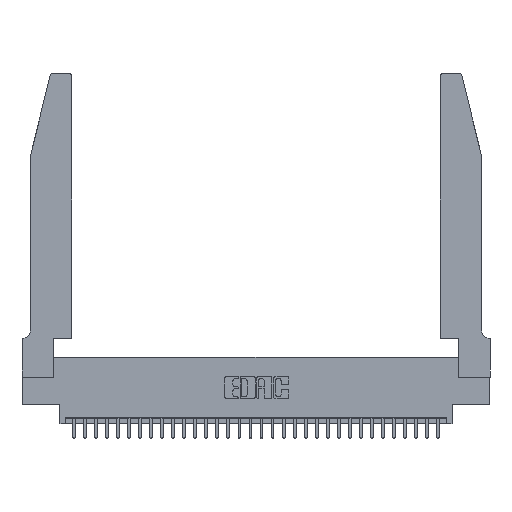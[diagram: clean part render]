
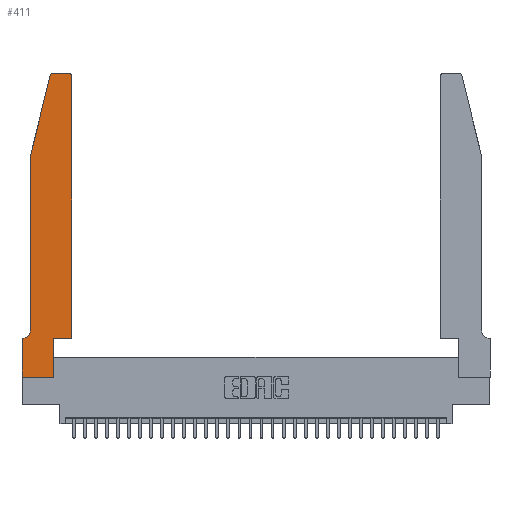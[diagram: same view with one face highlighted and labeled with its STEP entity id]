
A CAD part, top view. The second image highlights one B-rep face of the part: STEP entity #411.
In plain terms, the highlighted planar face has unit normal (0, 0, 1).
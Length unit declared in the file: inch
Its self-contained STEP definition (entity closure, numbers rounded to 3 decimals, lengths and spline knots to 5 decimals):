
#38 = ORIENTED_EDGE ( 'NONE', *, *, #1586, .T. ) ;
#411 = ADVANCED_FACE ( 'NONE', ( #4819 ), #22906, .T. ) ;
#814 = VERTEX_POINT ( 'NONE', #14764 ) ;
#944 = VECTOR ( 'NONE', #4393, 39.37008 ) ;
#1363 = CARTESIAN_POINT ( 'NONE',  ( 0., 0., 0.37 ) ) ;
#1586 = EDGE_CURVE ( 'NONE', #8249, #31456, #18300, .T. ) ;
#1672 = LINE ( 'NONE', #8475, #20260 ) ;
#2042 = ORIENTED_EDGE ( 'NONE', *, *, #30011, .T. ) ;
#2322 = CARTESIAN_POINT ( 'NONE',  ( 0.0055, 0.42, 0.37 ) ) ;
#2720 = CARTESIAN_POINT ( 'NONE',  ( 0.4505, 0.35, 0.37 ) ) ;
#2846 = ORIENTED_EDGE ( 'NONE', *, *, #5750, .T. ) ;
#3262 = ORIENTED_EDGE ( 'NONE', *, *, #23951, .T. ) ;
#3303 = VERTEX_POINT ( 'NONE', #9150 ) ;
#3480 = DIRECTION ( 'NONE',  ( 0., 1., 0. ) ) ;
#3857 = VECTOR ( 'NONE', #28769, 39.37008 ) ;
#3922 = DIRECTION ( 'NONE',  ( 0., -1., 0. ) ) ;
#4048 = ORIENTED_EDGE ( 'NONE', *, *, #29723, .T. ) ;
#4266 = AXIS2_PLACEMENT_3D ( 'NONE', #14366, #31878, #16881 ) ;
#4328 = VECTOR ( 'NONE', #3480, 39.37008 ) ;
#4393 = DIRECTION ( 'NONE',  ( 1., 0., 0. ) ) ;
#4819 = FACE_OUTER_BOUND ( 'NONE', #18458, .T. ) ;
#4869 = DIRECTION ( 'NONE',  ( -1., 0., 0. ) ) ;
#5144 = LINE ( 'NONE', #1363, #11954 ) ;
#5384 = EDGE_CURVE ( 'NONE', #3303, #18083, #32513, .T. ) ;
#5750 = EDGE_CURVE ( 'NONE', #12288, #8249, #10564, .T. ) ;
#6104 = CARTESIAN_POINT ( 'NONE',  ( 0., 0., 0.37 ) ) ;
#6639 = CARTESIAN_POINT ( 'NONE',  ( 0.2865, 0., 0.37 ) ) ;
#6648 = CARTESIAN_POINT ( 'NONE',  ( 0.0755, 0.35, 0.37 ) ) ;
#7475 = CARTESIAN_POINT ( 'NONE',  ( 0.284, 2.72, 0.37 ) ) ;
#7610 = VECTOR ( 'NONE', #21838, 39.37008 ) ;
#7743 = LINE ( 'NONE', #19524, #944 ) ;
#8249 = VERTEX_POINT ( 'NONE', #21257 ) ;
#8399 = LINE ( 'NONE', #6648, #7610 ) ;
#8475 = CARTESIAN_POINT ( 'NONE',  ( 0.2605, 2.75, 0.37 ) ) ;
#8563 = AXIS2_PLACEMENT_3D ( 'NONE', #7475, #25084, #10050 ) ;
#9035 = CARTESIAN_POINT ( 'NONE',  ( 0.4205, 2.75, 0.37 ) ) ;
#9063 = EDGE_CURVE ( 'NONE', #814, #18922, #18988, .T. ) ;
#9150 = CARTESIAN_POINT ( 'NONE',  ( 0.4505, 0.35, 0.37 ) ) ;
#9441 = LINE ( 'NONE', #22364, #11059 ) ;
#10050 = DIRECTION ( 'NONE',  ( 1., 0., 0. ) ) ;
#10564 = LINE ( 'NONE', #24123, #29731 ) ;
#10601 = VERTEX_POINT ( 'NONE', #6639 ) ;
#11059 = VECTOR ( 'NONE', #24932, 39.37008 ) ;
#11954 = VECTOR ( 'NONE', #29141, 39.37008 ) ;
#12288 = VERTEX_POINT ( 'NONE', #15922 ) ;
#13344 = VECTOR ( 'NONE', #17918, 39.37008 ) ;
#13607 = ORIENTED_EDGE ( 'NONE', *, *, #23360, .T. ) ;
#13981 = ORIENTED_EDGE ( 'NONE', *, *, #9063, .T. ) ;
#13996 = CARTESIAN_POINT ( 'NONE',  ( 0.4505, 2.72, 0.37 ) ) ;
#14155 = VERTEX_POINT ( 'NONE', #14190 ) ;
#14190 = CARTESIAN_POINT ( 'NONE',  ( 0., 0.35, 0.37 ) ) ;
#14366 = CARTESIAN_POINT ( 'NONE',  ( 0.4205, 2.72, 0.37 ) ) ;
#14764 = CARTESIAN_POINT ( 'NONE',  ( 0.284, 2.75, 0.37 ) ) ;
#15562 = ORIENTED_EDGE ( 'NONE', *, *, #19758, .T. ) ;
#15625 = AXIS2_PLACEMENT_3D ( 'NONE', #2322, #20011, #4869 ) ;
#15922 = CARTESIAN_POINT ( 'NONE',  ( 0.0755, 2., 0.37 ) ) ;
#16015 = VERTEX_POINT ( 'NONE', #28759 ) ;
#16089 = DIRECTION ( 'NONE',  ( -1., 0., 0. ) ) ;
#16842 = EDGE_CURVE ( 'NONE', #16015, #3303, #7743, .T. ) ;
#16881 = DIRECTION ( 'NONE',  ( 1., 0., 0. ) ) ;
#17330 = LINE ( 'NONE', #6104, #3857 ) ;
#17918 = DIRECTION ( 'NONE',  ( 0., 1., 0. ) ) ;
#18083 = VERTEX_POINT ( 'NONE', #13996 ) ;
#18300 = CIRCLE ( 'NONE', #15625, 0.07 ) ;
#18363 = ORIENTED_EDGE ( 'NONE', *, *, #5384, .T. ) ;
#18458 = EDGE_LOOP ( 'NONE', ( #26886, #13981, #2042, #2846, #38, #13607, #3262, #4048, #15562, #28899, #18363, #25811 ) ) ;
#18567 = DIRECTION ( 'NONE',  ( 1., 0., 0. ) ) ;
#18648 = CARTESIAN_POINT ( 'NONE',  ( 0.2865, 0.35, 0.37 ) ) ;
#18922 = VERTEX_POINT ( 'NONE', #27846 ) ;
#18952 = VERTEX_POINT ( 'NONE', #22902 ) ;
#18988 = CIRCLE ( 'NONE', #8563, 0.03 ) ;
#19524 = CARTESIAN_POINT ( 'NONE',  ( 0.4505, 0.35, 0.37 ) ) ;
#19758 = EDGE_CURVE ( 'NONE', #10601, #16015, #31110, .T. ) ;
#19877 = CARTESIAN_POINT ( 'NONE',  ( 0., 0.35, 0.37 ) ) ;
#20011 = DIRECTION ( 'NONE',  ( 0., 0., -1. ) ) ;
#20260 = VECTOR ( 'NONE', #16089, 39.37008 ) ;
#20861 = AXIS2_PLACEMENT_3D ( 'NONE', #19877, #26525, #18567 ) ;
#21257 = CARTESIAN_POINT ( 'NONE',  ( 0.0755, 0.42, 0.37 ) ) ;
#21838 = DIRECTION ( 'NONE',  ( -1., 0., 0. ) ) ;
#22364 = CARTESIAN_POINT ( 'NONE',  ( 0.0755, 2., 0.37 ) ) ;
#22424 = EDGE_CURVE ( 'NONE', #30726, #814, #1672, .T. ) ;
#22902 = CARTESIAN_POINT ( 'NONE',  ( 0., 0., 0.37 ) ) ;
#22906 = PLANE ( 'NONE',  #20861 ) ;
#23360 = EDGE_CURVE ( 'NONE', #31456, #14155, #8399, .T. ) ;
#23702 = CIRCLE ( 'NONE', #4266, 0.03 ) ;
#23951 = EDGE_CURVE ( 'NONE', #14155, #18952, #5144, .T. ) ;
#24041 = EDGE_CURVE ( 'NONE', #18083, #30726, #23702, .T. ) ;
#24123 = CARTESIAN_POINT ( 'NONE',  ( 0.0755, 2., 0.37 ) ) ;
#24592 = CARTESIAN_POINT ( 'NONE',  ( 0.0055, 0.35, 0.37 ) ) ;
#24932 = DIRECTION ( 'NONE',  ( -0.239, -0.971, 0. ) ) ;
#25084 = DIRECTION ( 'NONE',  ( 0., 0., 1. ) ) ;
#25811 = ORIENTED_EDGE ( 'NONE', *, *, #24041, .T. ) ;
#26525 = DIRECTION ( 'NONE',  ( 0., 0., 1. ) ) ;
#26886 = ORIENTED_EDGE ( 'NONE', *, *, #22424, .T. ) ;
#27846 = CARTESIAN_POINT ( 'NONE',  ( 0.25487, 2.72718, 0.37 ) ) ;
#28759 = CARTESIAN_POINT ( 'NONE',  ( 0.2865, 0.35, 0.37 ) ) ;
#28769 = DIRECTION ( 'NONE',  ( 1., 0., 0. ) ) ;
#28899 = ORIENTED_EDGE ( 'NONE', *, *, #16842, .T. ) ;
#29141 = DIRECTION ( 'NONE',  ( 0., -1., 0. ) ) ;
#29723 = EDGE_CURVE ( 'NONE', #18952, #10601, #17330, .T. ) ;
#29731 = VECTOR ( 'NONE', #3922, 39.37008 ) ;
#30011 = EDGE_CURVE ( 'NONE', #18922, #12288, #9441, .T. ) ;
#30726 = VERTEX_POINT ( 'NONE', #9035 ) ;
#31110 = LINE ( 'NONE', #18648, #4328 ) ;
#31456 = VERTEX_POINT ( 'NONE', #24592 ) ;
#31878 = DIRECTION ( 'NONE',  ( 0., 0., 1. ) ) ;
#32513 = LINE ( 'NONE', #2720, #13344 ) ;
